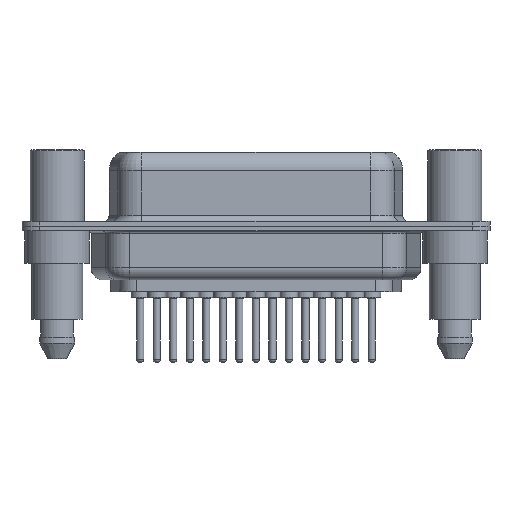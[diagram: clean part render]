
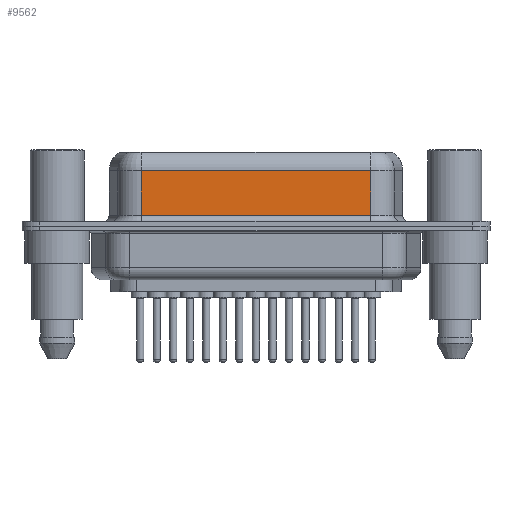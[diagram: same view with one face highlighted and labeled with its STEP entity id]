
A CAD part, front view. The second image highlights one B-rep face of the part: STEP entity #9562.
In plain terms, the highlighted planar face has unit normal (0, -1, 0).
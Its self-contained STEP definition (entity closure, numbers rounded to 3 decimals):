
#327 = CARTESIAN_POINT ( 'NONE',  ( 7.038, -3.95, 6.4 ) ) ;
#1736 = VECTOR ( 'NONE', #13084, 1000. ) ;
#2187 = VECTOR ( 'NONE', #18256, 1000. ) ;
#2440 = EDGE_LOOP ( 'NONE', ( #17620, #9238, #2662, #12659 ) ) ;
#2553 = CARTESIAN_POINT ( 'NONE',  ( 26.262, -3.95, 4.65 ) ) ;
#2662 = ORIENTED_EDGE ( 'NONE', *, *, #14300, .T. ) ;
#3053 = VECTOR ( 'NONE', #17280, 1000. ) ;
#3417 = CARTESIAN_POINT ( 'NONE',  ( 26.262, -3.95, 6.4 ) ) ;
#3763 = AXIS2_PLACEMENT_3D ( 'NONE', #7416, #4650, #11571 ) ;
#4650 = DIRECTION ( 'NONE',  ( 0., 1., 0. ) ) ;
#5141 = VERTEX_POINT ( 'NONE', #13961 ) ;
#5965 = LINE ( 'NONE', #11775, #1736 ) ;
#7416 = CARTESIAN_POINT ( 'NONE',  ( 26.262, -3.95, 6.4 ) ) ;
#8350 = EDGE_CURVE ( 'NONE', #16190, #12424, #8679, .T. ) ;
#8679 = LINE ( 'NONE', #3417, #3053 ) ;
#9238 = ORIENTED_EDGE ( 'NONE', *, *, #14995, .T. ) ;
#9562 = ADVANCED_FACE ( 'NONE', ( #13147 ), #15836, .F. ) ;
#10446 = EDGE_CURVE ( 'NONE', #12526, #12424, #5965, .T. ) ;
#11569 = LINE ( 'NONE', #327, #2187 ) ;
#11570 = CARTESIAN_POINT ( 'NONE',  ( 26.262, -3.95, 0.9 ) ) ;
#11571 = DIRECTION ( 'NONE',  ( -1., 0., 0. ) ) ;
#11775 = CARTESIAN_POINT ( 'NONE',  ( 26.262, -3.95, 0.9 ) ) ;
#12424 = VERTEX_POINT ( 'NONE', #11570 ) ;
#12526 = VERTEX_POINT ( 'NONE', #15478 ) ;
#12659 = ORIENTED_EDGE ( 'NONE', *, *, #10446, .T. ) ;
#12697 = VECTOR ( 'NONE', #17402, 1000. ) ;
#13084 = DIRECTION ( 'NONE',  ( 1., 0., 0. ) ) ;
#13147 = FACE_OUTER_BOUND ( 'NONE', #2440, .T. ) ;
#13961 = CARTESIAN_POINT ( 'NONE',  ( 7.038, -3.95, 4.65 ) ) ;
#14300 = EDGE_CURVE ( 'NONE', #5141, #12526, #11569, .T. ) ;
#14995 = EDGE_CURVE ( 'NONE', #16190, #5141, #15197, .T. ) ;
#15197 = LINE ( 'NONE', #2553, #12697 ) ;
#15478 = CARTESIAN_POINT ( 'NONE',  ( 7.038, -3.95, 0.9 ) ) ;
#15836 = PLANE ( 'NONE',  #3763 ) ;
#16158 = CARTESIAN_POINT ( 'NONE',  ( 26.262, -3.95, 4.65 ) ) ;
#16190 = VERTEX_POINT ( 'NONE', #16158 ) ;
#17280 = DIRECTION ( 'NONE',  ( 0., 0., -1. ) ) ;
#17402 = DIRECTION ( 'NONE',  ( -1., 0., 0. ) ) ;
#17620 = ORIENTED_EDGE ( 'NONE', *, *, #8350, .F. ) ;
#18256 = DIRECTION ( 'NONE',  ( 0., 0., -1. ) ) ;
